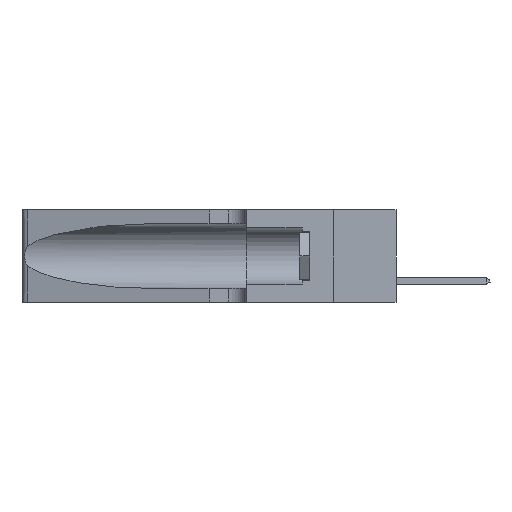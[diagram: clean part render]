
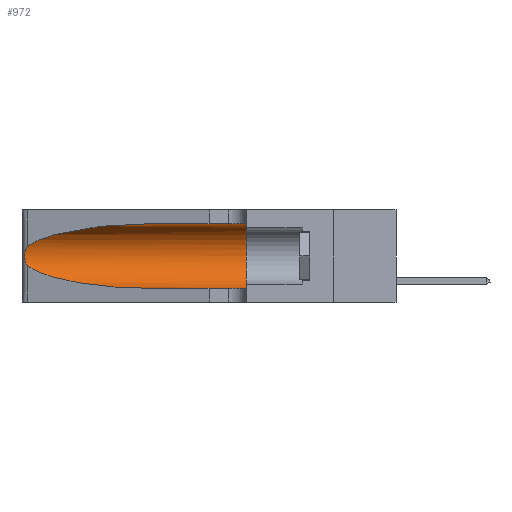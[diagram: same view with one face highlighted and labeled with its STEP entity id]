
A CAD part, left-side view. The second image highlights one B-rep face of the part: STEP entity #972.
In plain terms, the highlighted cylindrical face has radius 3.308 mm (diameter 6.617 mm), a partial arc.
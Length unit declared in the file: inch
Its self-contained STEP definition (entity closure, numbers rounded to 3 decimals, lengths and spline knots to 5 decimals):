
#112 = CARTESIAN_POINT ( 'NONE',  ( 0.25856, 1.23593, 0.16098 ) ) ;
#126 = CARTESIAN_POINT ( 'NONE',  ( 0.25487, 1.22718, 0.22369 ) ) ;
#623 = VERTEX_POINT ( 'NONE', #8599 ) ;
#972 = ADVANCED_FACE ( 'NONE', ( #11658 ), #10258, .F. ) ;
#1066 = CARTESIAN_POINT ( 'NONE',  ( 0.1305, 0.35, 0.05475 ) ) ;
#1399 =( BOUNDED_CURVE ( )  B_SPLINE_CURVE ( 3, ( #11696, #14598, #13254, #2409 ),
 .UNSPECIFIED., .F., .T. ) 
 B_SPLINE_CURVE_WITH_KNOTS ( ( 4, 4 ),
 ( 1.5708, 2.84003 ),
 .UNSPECIFIED. ) 
 CURVE ( )  GEOMETRIC_REPRESENTATION_ITEM ( )  RATIONAL_B_SPLINE_CURVE ( ( 1., 0.87, 0.87, 1. ) ) 
 REPRESENTATION_ITEM ( '' )  );
#1429 = CARTESIAN_POINT ( 'NONE',  ( 0.25487, 1.22718, 0.22369 ) ) ;
#1496 = VECTOR ( 'NONE', #4591, 39.37008 ) ;
#1875 = CARTESIAN_POINT ( 'NONE',  ( 0.26075, 1.23896, 0.178 ) ) ;
#1965 = CARTESIAN_POINT ( 'NONE',  ( 0.1305, 0.35, 0.185 ) ) ;
#2240 = VERTEX_POINT ( 'NONE', #18068 ) ;
#2409 = CARTESIAN_POINT ( 'NONE',  ( 0.25487, 1.22718, 0.22369 ) ) ;
#2423 = CARTESIAN_POINT ( 'NONE',  ( 0.18966, 0.96281, 0.05475 ) ) ;
#2485 = ORIENTED_EDGE ( 'NONE', *, *, #2566, .T. ) ;
#2566 = EDGE_CURVE ( 'NONE', #623, #18084, #8643, .T. ) ;
#2722 = EDGE_CURVE ( 'NONE', #6415, #19367, #1399, .T. ) ;
#3276 = CARTESIAN_POINT ( 'NONE',  ( 0.25789, 1.23486, 0.15765 ) ) ;
#4052 = ORIENTED_EDGE ( 'NONE', *, *, #2722, .T. ) ;
#4068 = CARTESIAN_POINT ( 'NONE',  ( 0.1305, 0.72297, 0.31525 ) ) ;
#4107 = DIRECTION ( 'NONE',  ( 0., -1., 0. ) ) ;
#4192 = ORIENTED_EDGE ( 'NONE', *, *, #5909, .T. ) ;
#4591 = DIRECTION ( 'NONE',  ( 0., -1., 0. ) ) ;
#4897 = B_SPLINE_CURVE_WITH_KNOTS ( 'NONE', 3,
 ( #1429, #13619, #13538, #10540, #12238, #10917, #16916, #1875, #6384, #112, #3276, #16783, #9416, #16987 ),
 .UNSPECIFIED., .F., .F.,
 ( 4, 2, 2, 2, 2, 2, 4 ),
 ( 0., 0.00027, 0.00053, 0.00107, 0.0016, 0.00187, 0.00214 ),
 .UNSPECIFIED. ) ;
#5909 = EDGE_CURVE ( 'NONE', #19367, #623, #4897, .T. ) ;
#6384 = CARTESIAN_POINT ( 'NONE',  ( 0.26017, 1.23833, 0.17102 ) ) ;
#6415 = VERTEX_POINT ( 'NONE', #4068 ) ;
#6493 = ORIENTED_EDGE ( 'NONE', *, *, #15483, .F. ) ;
#6648 = DIRECTION ( 'NONE',  ( 0., 0., 1. ) ) ;
#6930 = CARTESIAN_POINT ( 'NONE',  ( 0.1305, 1.61858, 0.05475 ) ) ;
#7034 = CARTESIAN_POINT ( 'NONE',  ( 0.2373, 1.15595, 0.08982 ) ) ;
#7060 = CARTESIAN_POINT ( 'NONE',  ( 0.1305, 1.61858, 0.185 ) ) ;
#8031 = DIRECTION ( 'NONE',  ( 0., 1., 0. ) ) ;
#8221 = EDGE_LOOP ( 'NONE', ( #4052, #4192, #2485, #15158, #9602, #6493 ) ) ;
#8599 = CARTESIAN_POINT ( 'NONE',  ( 0.25487, 1.22718, 0.14631 ) ) ;
#8643 =( BOUNDED_CURVE ( )  B_SPLINE_CURVE ( 3, ( #13069, #7034, #2423, #17676 ),
 .UNSPECIFIED., .F., .T. ) 
 B_SPLINE_CURVE_WITH_KNOTS ( ( 4, 4 ),
 ( 3.44316, 4.71239 ),
 .UNSPECIFIED. ) 
 CURVE ( )  GEOMETRIC_REPRESENTATION_ITEM ( )  RATIONAL_B_SPLINE_CURVE ( ( 1., 0.87, 0.87, 1. ) ) 
 REPRESENTATION_ITEM ( '' )  );
#8716 = VERTEX_POINT ( 'NONE', #1066 ) ;
#9003 = LINE ( 'NONE', #6930, #14945 ) ;
#9416 = CARTESIAN_POINT ( 'NONE',  ( 0.25555, 1.22993, 0.14849 ) ) ;
#9602 = ORIENTED_EDGE ( 'NONE', *, *, #19475, .F. ) ;
#10090 = CIRCLE ( 'NONE', #15291, 0.13025 ) ;
#10258 = CYLINDRICAL_SURFACE ( 'NONE', #12364, 0.13025 ) ;
#10371 = EDGE_CURVE ( 'NONE', #18084, #8716, #9003, .T. ) ;
#10540 = CARTESIAN_POINT ( 'NONE',  ( 0.25787, 1.23484, 0.2124 ) ) ;
#10917 = CARTESIAN_POINT ( 'NONE',  ( 0.26018, 1.23835, 0.19895 ) ) ;
#11658 = FACE_OUTER_BOUND ( 'NONE', #8221, .T. ) ;
#11696 = CARTESIAN_POINT ( 'NONE',  ( 0.1305, 0.72297, 0.31525 ) ) ;
#11849 = DIRECTION ( 'NONE',  ( 0., 0., -1. ) ) ;
#12238 = CARTESIAN_POINT ( 'NONE',  ( 0.25854, 1.2359, 0.20912 ) ) ;
#12240 = DIRECTION ( 'NONE',  ( 0., -1., 0. ) ) ;
#12364 = AXIS2_PLACEMENT_3D ( 'NONE', #7060, #4107, #11849 ) ;
#12597 = LINE ( 'NONE', #16214, #1496 ) ;
#13069 = CARTESIAN_POINT ( 'NONE',  ( 0.25487, 1.22718, 0.14631 ) ) ;
#13254 = CARTESIAN_POINT ( 'NONE',  ( 0.2373, 1.15595, 0.28018 ) ) ;
#13538 = CARTESIAN_POINT ( 'NONE',  ( 0.25639, 1.23184, 0.21858 ) ) ;
#13619 = CARTESIAN_POINT ( 'NONE',  ( 0.25555, 1.22994, 0.2215 ) ) ;
#14598 = CARTESIAN_POINT ( 'NONE',  ( 0.18966, 0.96281, 0.31525 ) ) ;
#14945 = VECTOR ( 'NONE', #12240, 39.37008 ) ;
#15158 = ORIENTED_EDGE ( 'NONE', *, *, #10371, .T. ) ;
#15291 = AXIS2_PLACEMENT_3D ( 'NONE', #1965, #8031, #6648 ) ;
#15483 = EDGE_CURVE ( 'NONE', #6415, #2240, #12597, .T. ) ;
#16214 = CARTESIAN_POINT ( 'NONE',  ( 0.1305, 1.61858, 0.31525 ) ) ;
#16783 = CARTESIAN_POINT ( 'NONE',  ( 0.25639, 1.23186, 0.15144 ) ) ;
#16916 = CARTESIAN_POINT ( 'NONE',  ( 0.26075, 1.23896, 0.19203 ) ) ;
#16987 = CARTESIAN_POINT ( 'NONE',  ( 0.25487, 1.22718, 0.14631 ) ) ;
#17676 = CARTESIAN_POINT ( 'NONE',  ( 0.1305, 0.72297, 0.05475 ) ) ;
#17980 = CARTESIAN_POINT ( 'NONE',  ( 0.1305, 0.72297, 0.05475 ) ) ;
#18068 = CARTESIAN_POINT ( 'NONE',  ( 0.1305, 0.35, 0.31525 ) ) ;
#18084 = VERTEX_POINT ( 'NONE', #17980 ) ;
#19367 = VERTEX_POINT ( 'NONE', #126 ) ;
#19475 = EDGE_CURVE ( 'NONE', #2240, #8716, #10090, .T. ) ;
